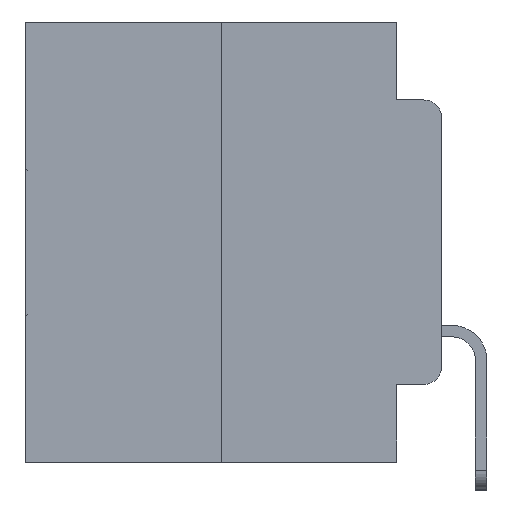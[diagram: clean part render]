
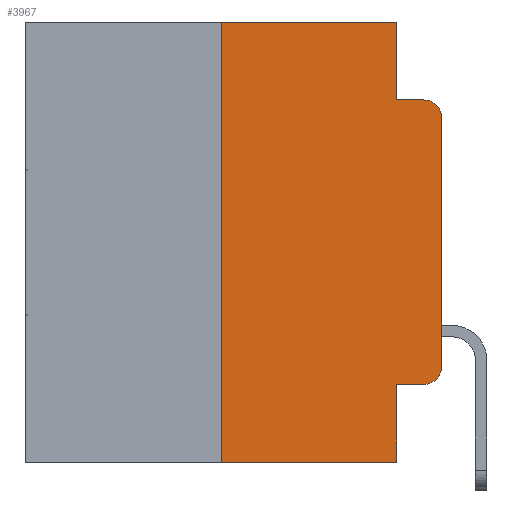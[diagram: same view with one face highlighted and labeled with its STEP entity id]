
A CAD part, left-side view. The second image highlights one B-rep face of the part: STEP entity #3967.
In plain terms, the highlighted planar face has unit normal (-1, 0, 0).
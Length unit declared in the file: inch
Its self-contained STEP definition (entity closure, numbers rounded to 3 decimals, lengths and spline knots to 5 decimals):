
#247 = VERTEX_POINT ( 'NONE', #24970 ) ;
#470 = CARTESIAN_POINT ( 'NONE',  ( 0., 0.051, -0.5 ) ) ;
#971 = CARTESIAN_POINT ( 'NONE',  ( 0., 0., 0. ) ) ;
#1561 = PLANE ( 'NONE',  #25528 ) ;
#1755 = AXIS2_PLACEMENT_3D ( 'NONE', #23733, #10864, #25734 ) ;
#1782 = DIRECTION ( 'NONE',  ( 0., -1., 0. ) ) ;
#2030 = VECTOR ( 'NONE', #14848, 39.37008 ) ;
#2222 = ORIENTED_EDGE ( 'NONE', *, *, #11330, .T. ) ;
#3822 = VERTEX_POINT ( 'NONE', #470 ) ;
#3851 = VERTEX_POINT ( 'NONE', #17813 ) ;
#3937 = LINE ( 'NONE', #20281, #16039 ) ;
#3967 = ADVANCED_FACE ( 'NONE', ( #16444 ), #1561, .F. ) ;
#4015 = CARTESIAN_POINT ( 'NONE',  ( 0., 0.051, 0. ) ) ;
#4147 = ORIENTED_EDGE ( 'NONE', *, *, #26875, .T. ) ;
#4886 = VECTOR ( 'NONE', #20276, 39.37008 ) ;
#5087 = CARTESIAN_POINT ( 'NONE',  ( 0., 0.051, -0.0885 ) ) ;
#5115 = VECTOR ( 'NONE', #1782, 39.37008 ) ;
#5217 = CARTESIAN_POINT ( 'NONE',  ( 0., 0.051, -0.4115 ) ) ;
#5706 = CIRCLE ( 'NONE', #17098, 0.02 ) ;
#6022 = DIRECTION ( 'NONE',  ( 0., 0., 1. ) ) ;
#6155 = LINE ( 'NONE', #10898, #11929 ) ;
#6345 = ORIENTED_EDGE ( 'NONE', *, *, #22910, .F. ) ;
#6497 = ORIENTED_EDGE ( 'NONE', *, *, #9765, .T. ) ;
#6636 = DIRECTION ( 'NONE',  ( -1., 0., 0. ) ) ;
#6944 = DIRECTION ( 'NONE',  ( 1., 0., 0. ) ) ;
#7288 = ORIENTED_EDGE ( 'NONE', *, *, #20165, .F. ) ;
#7850 = VERTEX_POINT ( 'NONE', #24425 ) ;
#9333 = CARTESIAN_POINT ( 'NONE',  ( 0., 0.473, 0. ) ) ;
#9765 = EDGE_CURVE ( 'NONE', #247, #24376, #20617, .T. ) ;
#9874 = CARTESIAN_POINT ( 'NONE',  ( 0., 0.051, 0. ) ) ;
#9975 = EDGE_CURVE ( 'NONE', #17515, #7850, #3937, .T. ) ;
#10121 = ORIENTED_EDGE ( 'NONE', *, *, #9975, .F. ) ;
#10319 = VECTOR ( 'NONE', #13518, 39.37008 ) ;
#10537 = ORIENTED_EDGE ( 'NONE', *, *, #14857, .T. ) ;
#10655 = CARTESIAN_POINT ( 'NONE',  ( 0., 0., -0.3915 ) ) ;
#10864 = DIRECTION ( 'NONE',  ( -1., 0., 0. ) ) ;
#10898 = CARTESIAN_POINT ( 'NONE',  ( 0., 0.25, 0. ) ) ;
#11330 = EDGE_CURVE ( 'NONE', #22155, #247, #26513, .T. ) ;
#11561 = DIRECTION ( 'NONE',  ( 0., -1., 0. ) ) ;
#11929 = VECTOR ( 'NONE', #6022, 39.37008 ) ;
#12098 = VERTEX_POINT ( 'NONE', #20275 ) ;
#12255 = DIRECTION ( 'NONE',  ( 0., 0., -1. ) ) ;
#12848 = ORIENTED_EDGE ( 'NONE', *, *, #25566, .T. ) ;
#12917 = EDGE_CURVE ( 'NONE', #22155, #3822, #20406, .T. ) ;
#13518 = DIRECTION ( 'NONE',  ( 0., -1., 0. ) ) ;
#14146 = ORIENTED_EDGE ( 'NONE', *, *, #21541, .F. ) ;
#14377 = LINE ( 'NONE', #971, #24773 ) ;
#14848 = DIRECTION ( 'NONE',  ( 0., -1., 0. ) ) ;
#14857 = EDGE_CURVE ( 'NONE', #23630, #3822, #21284, .T. ) ;
#15271 = VERTEX_POINT ( 'NONE', #26833 ) ;
#15470 = LINE ( 'NONE', #4015, #4886 ) ;
#15836 = DIRECTION ( 'NONE',  ( 0., 0., 1. ) ) ;
#15955 = EDGE_LOOP ( 'NONE', ( #4147, #12848, #6345, #14146, #10121, #7288, #10537, #17159, #2222, #6497 ) ) ;
#16039 = VECTOR ( 'NONE', #11561, 39.37008 ) ;
#16444 = FACE_OUTER_BOUND ( 'NONE', #15955, .T. ) ;
#16883 = CARTESIAN_POINT ( 'NONE',  ( 0., 0.25, 0. ) ) ;
#17098 = AXIS2_PLACEMENT_3D ( 'NONE', #20264, #6636, #22319 ) ;
#17159 = ORIENTED_EDGE ( 'NONE', *, *, #12917, .F. ) ;
#17515 = VERTEX_POINT ( 'NONE', #16883 ) ;
#17813 = CARTESIAN_POINT ( 'NONE',  ( 0., 0., -0.1085 ) ) ;
#18623 = CARTESIAN_POINT ( 'NONE',  ( 0., 0.051, -0.4115 ) ) ;
#19797 = VECTOR ( 'NONE', #12255, 39.37008 ) ;
#20165 = EDGE_CURVE ( 'NONE', #23630, #17515, #6155, .T. ) ;
#20264 = CARTESIAN_POINT ( 'NONE',  ( 0., 0.02, -0.1085 ) ) ;
#20275 = CARTESIAN_POINT ( 'NONE',  ( 0., 0.051, -0.0885 ) ) ;
#20276 = DIRECTION ( 'NONE',  ( 0., 0., -1. ) ) ;
#20281 = CARTESIAN_POINT ( 'NONE',  ( 0., 0.473, 0. ) ) ;
#20406 = LINE ( 'NONE', #9874, #19797 ) ;
#20617 = CIRCLE ( 'NONE', #1755, 0.02 ) ;
#21284 = LINE ( 'NONE', #25985, #10319 ) ;
#21541 = EDGE_CURVE ( 'NONE', #7850, #12098, #15470, .T. ) ;
#22155 = VERTEX_POINT ( 'NONE', #5217 ) ;
#22319 = DIRECTION ( 'NONE',  ( 0., 0., -1. ) ) ;
#22557 = DIRECTION ( 'NONE',  ( 0., 0., -1. ) ) ;
#22910 = EDGE_CURVE ( 'NONE', #12098, #15271, #25527, .T. ) ;
#23630 = VERTEX_POINT ( 'NONE', #24337 ) ;
#23733 = CARTESIAN_POINT ( 'NONE',  ( 0., 0.02, -0.3915 ) ) ;
#24337 = CARTESIAN_POINT ( 'NONE',  ( 0., 0.25, -0.5 ) ) ;
#24376 = VERTEX_POINT ( 'NONE', #10655 ) ;
#24425 = CARTESIAN_POINT ( 'NONE',  ( 0., 0.051, 0. ) ) ;
#24773 = VECTOR ( 'NONE', #15836, 39.37008 ) ;
#24970 = CARTESIAN_POINT ( 'NONE',  ( 0., 0.02, -0.4115 ) ) ;
#25528 = AXIS2_PLACEMENT_3D ( 'NONE', #9333, #6944, #22557 ) ;
#25527 = LINE ( 'NONE', #5087, #2030 ) ;
#25566 = EDGE_CURVE ( 'NONE', #3851, #15271, #5706, .T. ) ;
#25734 = DIRECTION ( 'NONE',  ( 0., 0., -1. ) ) ;
#25985 = CARTESIAN_POINT ( 'NONE',  ( 0., 0.473, -0.5 ) ) ;
#26513 = LINE ( 'NONE', #18623, #5115 ) ;
#26833 = CARTESIAN_POINT ( 'NONE',  ( 0., 0.02, -0.0885 ) ) ;
#26875 = EDGE_CURVE ( 'NONE', #24376, #3851, #14377, .T. ) ;
